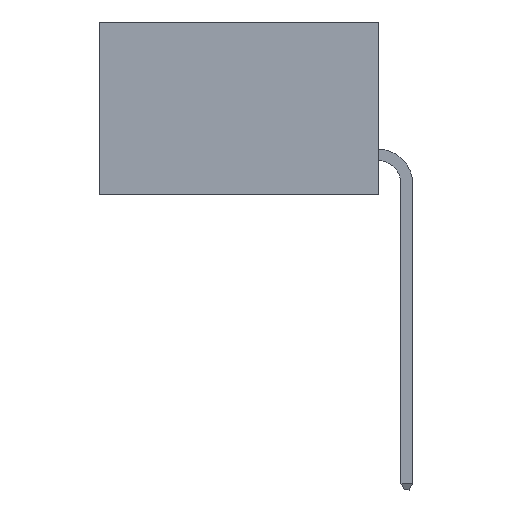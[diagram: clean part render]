
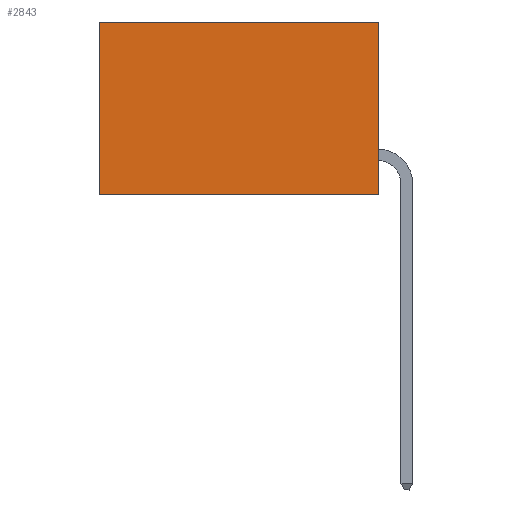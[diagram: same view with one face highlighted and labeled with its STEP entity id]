
A CAD part, left-side view. The second image highlights one B-rep face of the part: STEP entity #2843.
In plain terms, the highlighted planar face has unit normal (-1, 0, 0).
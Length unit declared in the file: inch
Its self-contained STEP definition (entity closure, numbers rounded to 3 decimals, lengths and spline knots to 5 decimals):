
#270 = DIRECTION ( 'NONE',  ( 0., 1., 0. ) ) ;
#380 = EDGE_LOOP ( 'NONE', ( #17917, #15716, #10548, #12290 ) ) ;
#743 = EDGE_CURVE ( 'NONE', #2814, #16206, #4924, .T. ) ;
#1805 = VERTEX_POINT ( 'NONE', #8745 ) ;
#2229 = PLANE ( 'NONE',  #6783 ) ;
#2814 = VERTEX_POINT ( 'NONE', #3474 ) ;
#2843 = ADVANCED_FACE ( 'NONE', ( #5754 ), #2229, .F. ) ;
#3080 = DIRECTION ( 'NONE',  ( 0., 1., 0. ) ) ;
#3344 = CARTESIAN_POINT ( 'NONE',  ( 0.298, 0.6, -0.37 ) ) ;
#3474 = CARTESIAN_POINT ( 'NONE',  ( 0.298, 0., -0.37 ) ) ;
#4047 = DIRECTION ( 'NONE',  ( 1., 0., 0. ) ) ;
#4089 = CARTESIAN_POINT ( 'NONE',  ( 0.298, 0., 0. ) ) ;
#4295 = DIRECTION ( 'NONE',  ( 0., 0., -1. ) ) ;
#4581 = CARTESIAN_POINT ( 'NONE',  ( 0.298, 0., -0.37 ) ) ;
#4924 = LINE ( 'NONE', #4581, #8321 ) ;
#5395 = CARTESIAN_POINT ( 'NONE',  ( 0.298, 0., 0. ) ) ;
#5483 = LINE ( 'NONE', #11291, #12623 ) ;
#5602 = LINE ( 'NONE', #15745, #12749 ) ;
#5754 = FACE_OUTER_BOUND ( 'NONE', #380, .T. ) ;
#6783 = AXIS2_PLACEMENT_3D ( 'NONE', #5395, #4047, #4295 ) ;
#7685 = EDGE_CURVE ( 'NONE', #18031, #1805, #5483, .T. ) ;
#7698 = LINE ( 'NONE', #4089, #17639 ) ;
#8321 = VECTOR ( 'NONE', #270, 39.37008 ) ;
#8745 = CARTESIAN_POINT ( 'NONE',  ( 0.298, 0.6, 0. ) ) ;
#9059 = EDGE_CURVE ( 'NONE', #18031, #2814, #7698, .T. ) ;
#9224 = CARTESIAN_POINT ( 'NONE',  ( 0.298, 0., 0. ) ) ;
#10548 = ORIENTED_EDGE ( 'NONE', *, *, #9059, .F. ) ;
#10644 = EDGE_CURVE ( 'NONE', #1805, #16206, #5602, .T. ) ;
#11291 = CARTESIAN_POINT ( 'NONE',  ( 0.298, 0., 0. ) ) ;
#12290 = ORIENTED_EDGE ( 'NONE', *, *, #7685, .T. ) ;
#12623 = VECTOR ( 'NONE', #3080, 39.37008 ) ;
#12749 = VECTOR ( 'NONE', #15706, 39.37008 ) ;
#12818 = DIRECTION ( 'NONE',  ( 0., 0., -1. ) ) ;
#15706 = DIRECTION ( 'NONE',  ( 0., 0., -1. ) ) ;
#15716 = ORIENTED_EDGE ( 'NONE', *, *, #743, .F. ) ;
#15745 = CARTESIAN_POINT ( 'NONE',  ( 0.298, 0.6, 0. ) ) ;
#16206 = VERTEX_POINT ( 'NONE', #3344 ) ;
#17639 = VECTOR ( 'NONE', #12818, 39.37008 ) ;
#17917 = ORIENTED_EDGE ( 'NONE', *, *, #10644, .T. ) ;
#18031 = VERTEX_POINT ( 'NONE', #9224 ) ;
